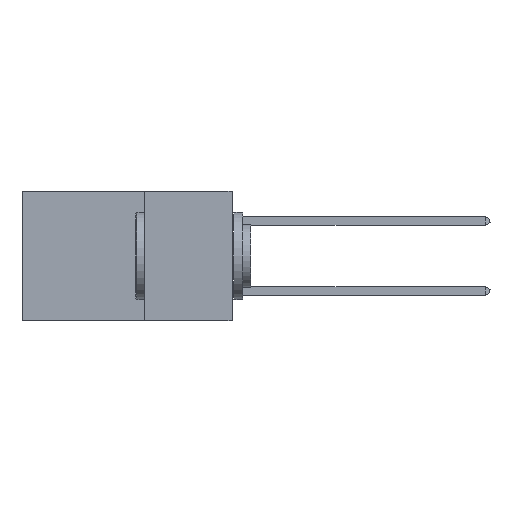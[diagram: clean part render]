
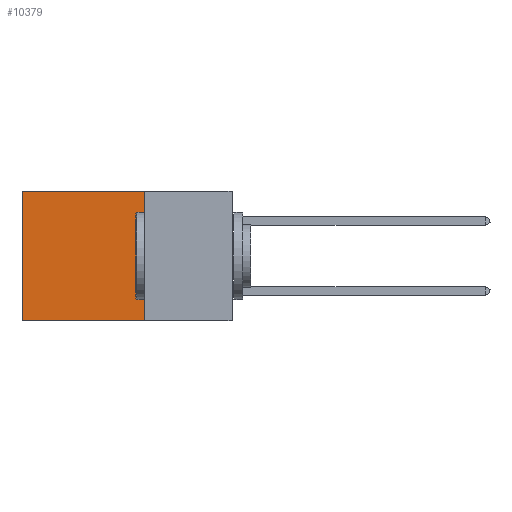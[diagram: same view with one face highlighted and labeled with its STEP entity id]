
A CAD part, left-side view. The second image highlights one B-rep face of the part: STEP entity #10379.
In plain terms, the highlighted planar face has unit normal (-1, 0, 0).
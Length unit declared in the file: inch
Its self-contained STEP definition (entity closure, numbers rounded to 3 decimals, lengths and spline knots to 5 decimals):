
#313 = VERTEX_POINT ( 'NONE', #14723 ) ;
#1030 = DIRECTION ( 'NONE',  ( 0., 1., 0. ) ) ;
#1167 = VECTOR ( 'NONE', #1030, 39.37008 ) ;
#1209 = FACE_OUTER_BOUND ( 'NONE', #16404, .T. ) ;
#3183 = DIRECTION ( 'NONE',  ( 1., 0., 0. ) ) ;
#3620 = EDGE_CURVE ( 'NONE', #8030, #313, #11335, .T. ) ;
#3787 = VERTEX_POINT ( 'NONE', #14097 ) ;
#3918 = DIRECTION ( 'NONE',  ( 0., 0., -1. ) ) ;
#3972 = VECTOR ( 'NONE', #15373, 39.37008 ) ;
#4253 = VERTEX_POINT ( 'NONE', #12373 ) ;
#5206 = CARTESIAN_POINT ( 'NONE',  ( 0.2875, 0.25, 0. ) ) ;
#6203 = CARTESIAN_POINT ( 'NONE',  ( 0.2875, 0.25, 0. ) ) ;
#7189 = LINE ( 'NONE', #12451, #10526 ) ;
#7503 = EDGE_CURVE ( 'NONE', #313, #3787, #7189, .T. ) ;
#8030 = VERTEX_POINT ( 'NONE', #5206 ) ;
#8891 = CARTESIAN_POINT ( 'NONE',  ( 0.2875, 0.25, 0. ) ) ;
#9139 = DIRECTION ( 'NONE',  ( 0., 0., -1. ) ) ;
#9177 = ORIENTED_EDGE ( 'NONE', *, *, #3620, .T. ) ;
#9790 = VECTOR ( 'NONE', #9139, 39.37008 ) ;
#10379 = ADVANCED_FACE ( 'NONE', ( #1209 ), #17207, .F. ) ;
#10526 = VECTOR ( 'NONE', #3918, 39.37008 ) ;
#11335 = LINE ( 'NONE', #14504, #1167 ) ;
#11927 = ORIENTED_EDGE ( 'NONE', *, *, #15364, .F. ) ;
#12055 = EDGE_CURVE ( 'NONE', #4253, #3787, #14882, .T. ) ;
#12250 = ORIENTED_EDGE ( 'NONE', *, *, #12055, .F. ) ;
#12373 = CARTESIAN_POINT ( 'NONE',  ( 0.2875, 0.25, -0.37 ) ) ;
#12451 = CARTESIAN_POINT ( 'NONE',  ( 0.2875, 0.6, 0. ) ) ;
#13153 = DIRECTION ( 'NONE',  ( 0., 0., -1. ) ) ;
#13537 = LINE ( 'NONE', #6203, #9790 ) ;
#13957 = CARTESIAN_POINT ( 'NONE',  ( 0.2875, 0.25, -0.37 ) ) ;
#14097 = CARTESIAN_POINT ( 'NONE',  ( 0.2875, 0.6, -0.37 ) ) ;
#14504 = CARTESIAN_POINT ( 'NONE',  ( 0.2875, 0.25, 0. ) ) ;
#14723 = CARTESIAN_POINT ( 'NONE',  ( 0.2875, 0.6, 0. ) ) ;
#14833 = AXIS2_PLACEMENT_3D ( 'NONE', #8891, #3183, #13153 ) ;
#14882 = LINE ( 'NONE', #13957, #3972 ) ;
#15364 = EDGE_CURVE ( 'NONE', #8030, #4253, #13537, .T. ) ;
#15373 = DIRECTION ( 'NONE',  ( 0., 1., 0. ) ) ;
#16404 = EDGE_LOOP ( 'NONE', ( #17668, #12250, #11927, #9177 ) ) ;
#17207 = PLANE ( 'NONE',  #14833 ) ;
#17668 = ORIENTED_EDGE ( 'NONE', *, *, #7503, .T. ) ;
